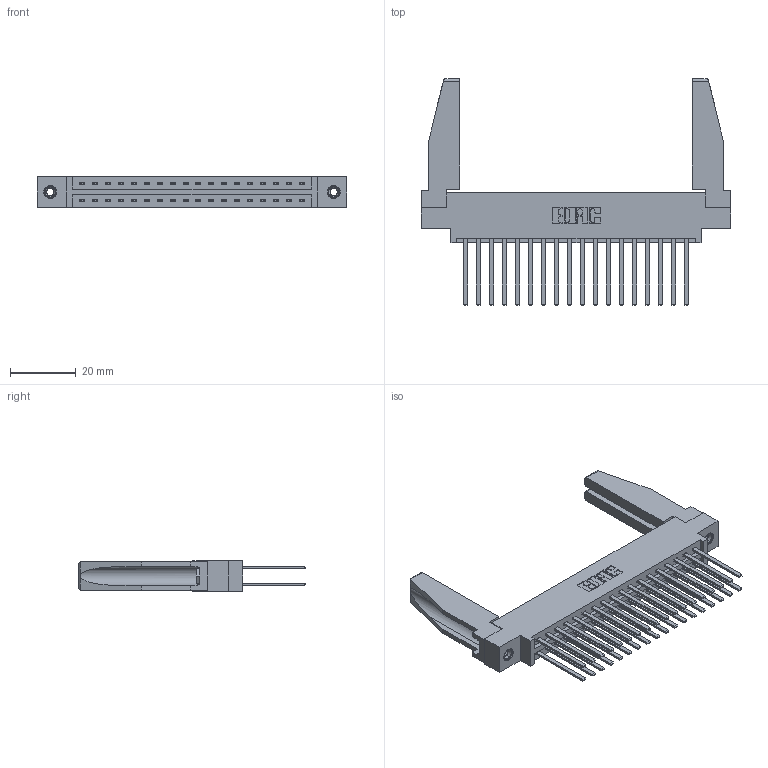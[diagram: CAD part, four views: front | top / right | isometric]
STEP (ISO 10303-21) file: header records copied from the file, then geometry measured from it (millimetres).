
FILE_DESCRIPTION (( 'STEP AP203' ), '1' );
FILE_NAME ('337-036-544-878.STEP', '2019-10-11T10:52:15', ( '' ), ( '' ), 'SwSTEP 2.0', 'SolidWorks 2016', '' );
FILE_SCHEMA (( 'CONFIG_CONTROL_DESIGN' ));
Length unit declared in the file: inch
Products named in the file (5): 337 Part_0.170 Offset - 0.156 Dia-TI; 337-036-544-878; 345-292-001_345-293-144; 345-250-001_345-250-001-102; 307-220-078
Assembly tree (41 placements, depth 2):
  337-036-544-878
    337 Part_0.170 Offset - 0.156 Dia-TI
    345-292-001_345-293-144  x36
    345-250-001_345-250-001-102  x2
    307-220-078  x2
Bounding box: 94.34 x 69.09 x 9.4 mm (x, y, z)
Volume: 14002.8 mm3; surface area: 16669.5 mm2
Topology: 41 solids, 41 shells, 1976 faces, 5801 edges, 3810 vertices
Faces by surface type: plane 1382, cylinder 578, cone 12, torus 4
Entity records: 19448 total; most frequent: CARTESIAN_POINT 3296, ORIENTED_EDGE 3188, DIRECTION 2850, EDGE_CURVE 1594, VECTOR 1432, LINE 1432, VERTEX_POINT 1056, AXIS2_PLACEMENT_3D 709
